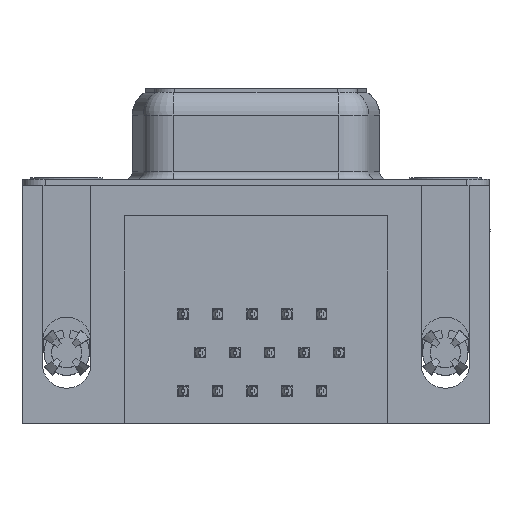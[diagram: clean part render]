
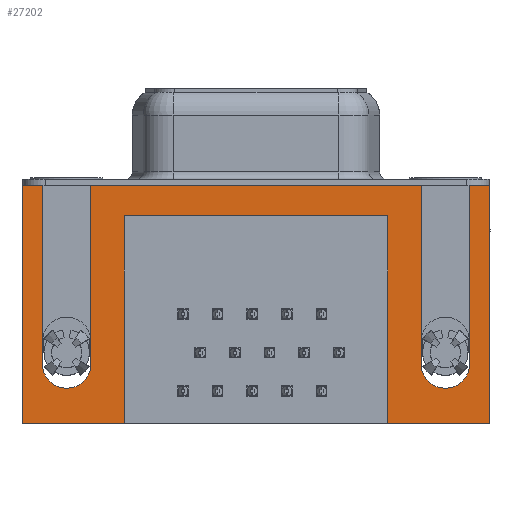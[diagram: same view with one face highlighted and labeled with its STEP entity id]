
A CAD part, front view. The second image highlights one B-rep face of the part: STEP entity #27202.
In plain terms, the highlighted planar face has unit normal (0, -1, 0).
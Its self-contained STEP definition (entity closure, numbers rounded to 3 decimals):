
#349 = CARTESIAN_POINT ( 'NONE',  ( 21.2, -6.275, -2. ) ) ;
#394 = DIRECTION ( 'NONE',  ( 0., 0., 1. ) ) ;
#425 = CARTESIAN_POINT ( 'NONE',  ( -1.6, -6.275, -11.78 ) ) ;
#472 = EDGE_CURVE ( 'NONE', #33864, #1633, #11592, .T. ) ;
#475 = CARTESIAN_POINT ( 'NONE',  ( 1.6, -6.275, -11.78 ) ) ;
#982 = LINE ( 'NONE', #3439, #23036 ) ;
#1633 = VERTEX_POINT ( 'NONE', #23309 ) ;
#1701 = EDGE_CURVE ( 'NONE', #32954, #13120, #33275, .T. ) ;
#1883 = DIRECTION ( 'NONE',  ( -1., 0., 0. ) ) ;
#1957 = DIRECTION ( 'NONE',  ( 0., -1., 0. ) ) ;
#2366 = CIRCLE ( 'NONE', #14049, 1.6 ) ;
#2428 = LINE ( 'NONE', #10457, #31916 ) ;
#3125 = CARTESIAN_POINT ( 'NONE',  ( -2.91, -6.275, -2.5 ) ) ;
#3414 = CARTESIAN_POINT ( 'NONE',  ( -1.6, -6.275, 0. ) ) ;
#3439 = CARTESIAN_POINT ( 'NONE',  ( 1.6, -6.275, 0. ) ) ;
#3796 = CARTESIAN_POINT ( 'NONE',  ( 27.9, -6.275, 0. ) ) ;
#4370 = ORIENTED_EDGE ( 'NONE', *, *, #1701, .F. ) ;
#4645 = LINE ( 'NONE', #20175, #26581 ) ;
#5361 = ORIENTED_EDGE ( 'NONE', *, *, #20480, .F. ) ;
#5390 = ORIENTED_EDGE ( 'NONE', *, *, #32166, .F. ) ;
#5888 = EDGE_CURVE ( 'NONE', #15988, #11041, #8082, .T. ) ;
#6044 = DIRECTION ( 'NONE',  ( 0., 0., -1. ) ) ;
#6172 = VERTEX_POINT ( 'NONE', #10287 ) ;
#6227 = EDGE_CURVE ( 'NONE', #36144, #9521, #17506, .T. ) ;
#6653 = FACE_OUTER_BOUND ( 'NONE', #22084, .T. ) ;
#6951 = ORIENTED_EDGE ( 'NONE', *, *, #17305, .F. ) ;
#7065 = CARTESIAN_POINT ( 'NONE',  ( 24.99, -6.275, -11.78 ) ) ;
#7711 = VERTEX_POINT ( 'NONE', #32976 ) ;
#8082 = LINE ( 'NONE', #8913, #13039 ) ;
#8369 = CARTESIAN_POINT ( 'NONE',  ( 3.79, -6.275, -2. ) ) ;
#8463 = ORIENTED_EDGE ( 'NONE', *, *, #472, .F. ) ;
#8625 = VERTEX_POINT ( 'NONE', #12945 ) ;
#8812 = CARTESIAN_POINT ( 'NONE',  ( 23.39, -6.275, 0. ) ) ;
#8816 = VECTOR ( 'NONE', #11995, 1000. ) ;
#8913 = CARTESIAN_POINT ( 'NONE',  ( 27.9, -6.275, -2.5 ) ) ;
#9516 = EDGE_CURVE ( 'NONE', #6172, #12664, #24046, .T. ) ;
#9521 = VERTEX_POINT ( 'NONE', #475 ) ;
#9956 = DIRECTION ( 'NONE',  ( -1., 0., 0. ) ) ;
#10266 = DIRECTION ( 'NONE',  ( 1., 0., 0. ) ) ;
#10287 = CARTESIAN_POINT ( 'NONE',  ( 21.2, -6.275, -15.7 ) ) ;
#10335 = VECTOR ( 'NONE', #10266, 1000. ) ;
#10457 = CARTESIAN_POINT ( 'NONE',  ( 27.9, -6.275, -15.7 ) ) ;
#11041 = VERTEX_POINT ( 'NONE', #3796 ) ;
#11235 = CARTESIAN_POINT ( 'NONE',  ( 27.9, -6.275, -15.7 ) ) ;
#11293 = DIRECTION ( 'NONE',  ( 1., 0., 0. ) ) ;
#11592 = LINE ( 'NONE', #8812, #33349 ) ;
#11777 = DIRECTION ( 'NONE',  ( 0., 0., -1. ) ) ;
#11805 = CARTESIAN_POINT ( 'NONE',  ( 3.79, -6.275, -15.7 ) ) ;
#11995 = DIRECTION ( 'NONE',  ( 0., 0., 1. ) ) ;
#12197 = ORIENTED_EDGE ( 'NONE', *, *, #6227, .F. ) ;
#12230 = CARTESIAN_POINT ( 'NONE',  ( -2.91, -6.275, -15.7 ) ) ;
#12349 = ORIENTED_EDGE ( 'NONE', *, *, #25532, .F. ) ;
#12605 = DIRECTION ( 'NONE',  ( -1., 0., 0. ) ) ;
#12664 = VERTEX_POINT ( 'NONE', #21879 ) ;
#12945 = CARTESIAN_POINT ( 'NONE',  ( 26.59, -6.275, -11.78 ) ) ;
#13039 = VECTOR ( 'NONE', #34536, 1000. ) ;
#13120 = VERTEX_POINT ( 'NONE', #29519 ) ;
#13313 = EDGE_CURVE ( 'NONE', #15988, #6172, #2428, .T. ) ;
#13539 = LINE ( 'NONE', #3414, #27774 ) ;
#14049 = AXIS2_PLACEMENT_3D ( 'NONE', #7065, #27066, #9956 ) ;
#14388 = ORIENTED_EDGE ( 'NONE', *, *, #24888, .F. ) ;
#15242 = EDGE_CURVE ( 'NONE', #21598, #11041, #4645, .T. ) ;
#15678 = ORIENTED_EDGE ( 'NONE', *, *, #36374, .F. ) ;
#15817 = CARTESIAN_POINT ( 'NONE',  ( -2.91, -6.275, 0. ) ) ;
#15988 = VERTEX_POINT ( 'NONE', #32943 ) ;
#16458 = VECTOR ( 'NONE', #28345, 1000. ) ;
#16682 = EDGE_CURVE ( 'NONE', #8625, #21598, #20287, .T. ) ;
#17077 = VECTOR ( 'NONE', #28296, 1000. ) ;
#17258 = ORIENTED_EDGE ( 'NONE', *, *, #25954, .F. ) ;
#17282 = ORIENTED_EDGE ( 'NONE', *, *, #16682, .F. ) ;
#17305 = EDGE_CURVE ( 'NONE', #24381, #36144, #13539, .T. ) ;
#17506 = CIRCLE ( 'NONE', #23829, 1.6 ) ;
#18313 = CARTESIAN_POINT ( 'NONE',  ( 26.59, -6.275, 0. ) ) ;
#18695 = CARTESIAN_POINT ( 'NONE',  ( 23.39, -6.275, 0. ) ) ;
#19202 = CARTESIAN_POINT ( 'NONE',  ( 0., -6.275, -11.78 ) ) ;
#20175 = CARTESIAN_POINT ( 'NONE',  ( -2.91, -6.275, 0. ) ) ;
#20287 = LINE ( 'NONE', #36751, #35324 ) ;
#20480 = EDGE_CURVE ( 'NONE', #13120, #24381, #25379, .T. ) ;
#20604 = DIRECTION ( 'NONE',  ( 0., 0., -1. ) ) ;
#21139 = LINE ( 'NONE', #29616, #36203 ) ;
#21415 = VERTEX_POINT ( 'NONE', #11805 ) ;
#21461 = LINE ( 'NONE', #11235, #28987 ) ;
#21598 = VERTEX_POINT ( 'NONE', #18313 ) ;
#21879 = CARTESIAN_POINT ( 'NONE',  ( 21.2, -6.275, -2. ) ) ;
#22040 = DIRECTION ( 'NONE',  ( 1., 0., 0. ) ) ;
#22084 = EDGE_LOOP ( 'NONE', ( #17282, #5390, #8463, #14388, #27579, #12197, #6951, #5361, #4370, #17258, #12349, #15678, #36734, #22589, #28591, #28984 ) ) ;
#22589 = ORIENTED_EDGE ( 'NONE', *, *, #13313, .F. ) ;
#22857 = CARTESIAN_POINT ( 'NONE',  ( 3.79, -6.275, -2. ) ) ;
#23036 = VECTOR ( 'NONE', #394, 1000. ) ;
#23226 = DIRECTION ( 'NONE',  ( 0., -1., 0. ) ) ;
#23309 = CARTESIAN_POINT ( 'NONE',  ( 23.39, -6.275, -11.78 ) ) ;
#23829 = AXIS2_PLACEMENT_3D ( 'NONE', #19202, #1957, #22040 ) ;
#24046 = LINE ( 'NONE', #349, #8816 ) ;
#24108 = VERTEX_POINT ( 'NONE', #22857 ) ;
#24381 = VERTEX_POINT ( 'NONE', #27153 ) ;
#24888 = EDGE_CURVE ( 'NONE', #7711, #33864, #33915, .T. ) ;
#25379 = LINE ( 'NONE', #25493, #31978 ) ;
#25493 = CARTESIAN_POINT ( 'NONE',  ( -2.91, -6.275, 0. ) ) ;
#25532 = EDGE_CURVE ( 'NONE', #24108, #21415, #32112, .T. ) ;
#25954 = EDGE_CURVE ( 'NONE', #21415, #32954, #21461, .T. ) ;
#26581 = VECTOR ( 'NONE', #11293, 1000. ) ;
#27066 = DIRECTION ( 'NONE',  ( 0., -1., 0. ) ) ;
#27153 = CARTESIAN_POINT ( 'NONE',  ( -1.6, -6.275, 0. ) ) ;
#27202 = ADVANCED_FACE ( 'NONE', ( #6653 ), #34434, .T. ) ;
#27277 = CARTESIAN_POINT ( 'NONE',  ( -2.91, -6.275, -2.5 ) ) ;
#27579 = ORIENTED_EDGE ( 'NONE', *, *, #35097, .F. ) ;
#27774 = VECTOR ( 'NONE', #20604, 1000. ) ;
#28256 = DIRECTION ( 'NONE',  ( -1., 0., 0. ) ) ;
#28296 = DIRECTION ( 'NONE',  ( 0., 0., -1. ) ) ;
#28345 = DIRECTION ( 'NONE',  ( 0., 0., 1. ) ) ;
#28591 = ORIENTED_EDGE ( 'NONE', *, *, #5888, .T. ) ;
#28984 = ORIENTED_EDGE ( 'NONE', *, *, #15242, .F. ) ;
#28987 = VECTOR ( 'NONE', #28256, 1000. ) ;
#29519 = CARTESIAN_POINT ( 'NONE',  ( -2.91, -6.275, 0. ) ) ;
#29616 = CARTESIAN_POINT ( 'NONE',  ( 3.79, -6.275, -2. ) ) ;
#31155 = DIRECTION ( 'NONE',  ( 1., 0., 0. ) ) ;
#31178 = AXIS2_PLACEMENT_3D ( 'NONE', #3125, #23226, #6044 ) ;
#31916 = VECTOR ( 'NONE', #1883, 1000. ) ;
#31978 = VECTOR ( 'NONE', #31155, 1000. ) ;
#32112 = LINE ( 'NONE', #8369, #17077 ) ;
#32166 = EDGE_CURVE ( 'NONE', #1633, #8625, #2366, .T. ) ;
#32943 = CARTESIAN_POINT ( 'NONE',  ( 27.9, -6.275, -15.7 ) ) ;
#32954 = VERTEX_POINT ( 'NONE', #12230 ) ;
#32976 = CARTESIAN_POINT ( 'NONE',  ( 1.6, -6.275, 0. ) ) ;
#33275 = LINE ( 'NONE', #27277, #16458 ) ;
#33349 = VECTOR ( 'NONE', #11777, 1000. ) ;
#33864 = VERTEX_POINT ( 'NONE', #18695 ) ;
#33868 = DIRECTION ( 'NONE',  ( 0., 0., 1. ) ) ;
#33915 = LINE ( 'NONE', #15817, #10335 ) ;
#34434 = PLANE ( 'NONE',  #31178 ) ;
#34536 = DIRECTION ( 'NONE',  ( 0., 0., 1. ) ) ;
#35097 = EDGE_CURVE ( 'NONE', #9521, #7711, #982, .T. ) ;
#35324 = VECTOR ( 'NONE', #33868, 1000. ) ;
#36144 = VERTEX_POINT ( 'NONE', #425 ) ;
#36203 = VECTOR ( 'NONE', #12605, 1000. ) ;
#36374 = EDGE_CURVE ( 'NONE', #12664, #24108, #21139, .T. ) ;
#36734 = ORIENTED_EDGE ( 'NONE', *, *, #9516, .F. ) ;
#36751 = CARTESIAN_POINT ( 'NONE',  ( 26.59, -6.275, 0. ) ) ;
